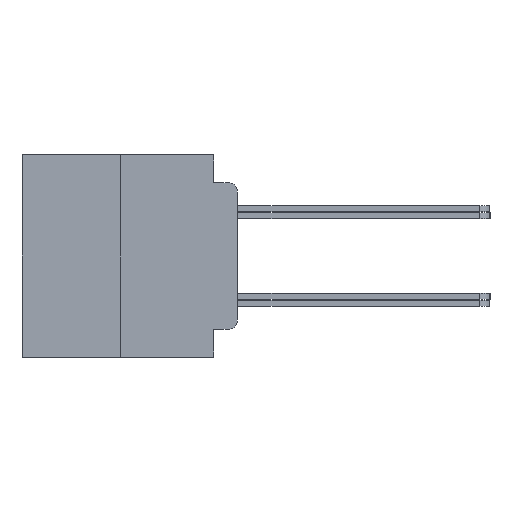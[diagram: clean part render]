
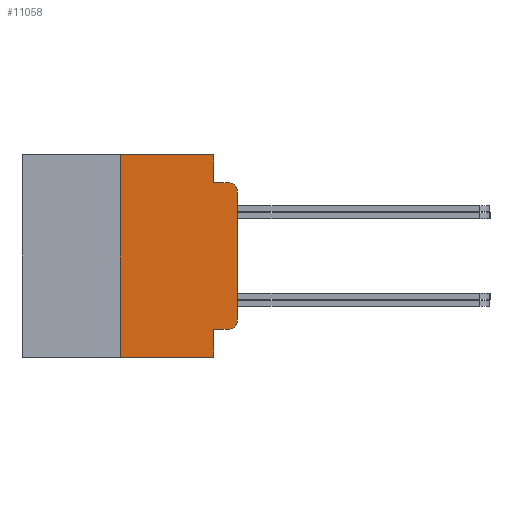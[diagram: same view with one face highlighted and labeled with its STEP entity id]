
A CAD part, left-side view. The second image highlights one B-rep face of the part: STEP entity #11058.
In plain terms, the highlighted planar face has unit normal (-1, 0, 0).
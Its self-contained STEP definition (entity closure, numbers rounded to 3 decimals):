
#409 = DIRECTION ( 'NONE',  ( 0., -1., 0. ) ) ;
#658 = VECTOR ( 'NONE', #10394, 1000. ) ;
#1171 = CARTESIAN_POINT ( 'NONE',  ( -75.603, 0.508, -3.975 ) ) ;
#1577 = PLANE ( 'NONE',  #27070 ) ;
#1828 = VERTEX_POINT ( 'NONE', #15472 ) ;
#2218 = CARTESIAN_POINT ( 'NONE',  ( -75.603, 0., -3.467 ) ) ;
#3144 = CARTESIAN_POINT ( 'NONE',  ( -75.603, 11.684, 5.486 ) ) ;
#3813 = DIRECTION ( 'NONE',  ( 0., 0., -1. ) ) ;
#3907 = DIRECTION ( 'NONE',  ( 1., 0., 0. ) ) ;
#4025 = VECTOR ( 'NONE', #7593, 1000. ) ;
#5191 = CARTESIAN_POINT ( 'NONE',  ( -75.603, 0.508, -3.467 ) ) ;
#5314 = EDGE_CURVE ( 'NONE', #27977, #28236, #26754, .T. ) ;
#5391 = FACE_OUTER_BOUND ( 'NONE', #5592, .T. ) ;
#5515 = EDGE_CURVE ( 'NONE', #28236, #13149, #27765, .T. ) ;
#5592 = EDGE_LOOP ( 'NONE', ( #6264, #5948, #16733, #16130, #12784, #23080, #10560, #15816, #26577, #27416 ) ) ;
#5948 = ORIENTED_EDGE ( 'NONE', *, *, #24408, .T. ) ;
#6264 = ORIENTED_EDGE ( 'NONE', *, *, #22663, .T. ) ;
#6413 = CARTESIAN_POINT ( 'NONE',  ( -75.603, 1.295, 5.486 ) ) ;
#6634 = LINE ( 'NONE', #12307, #8341 ) ;
#6705 = DIRECTION ( 'NONE',  ( 0., -1., 0. ) ) ;
#7097 = VERTEX_POINT ( 'NONE', #27868 ) ;
#7256 = CIRCLE ( 'NONE', #21825, 0.508 ) ;
#7593 = DIRECTION ( 'NONE',  ( 0., -1., 0. ) ) ;
#7601 = CIRCLE ( 'NONE', #17097, 0.508 ) ;
#8071 = CARTESIAN_POINT ( 'NONE',  ( -75.603, 1.295, -3.975 ) ) ;
#8266 = CARTESIAN_POINT ( 'NONE',  ( -75.603, 0.508, 3.467 ) ) ;
#8341 = VECTOR ( 'NONE', #18832, 1000. ) ;
#9638 = LINE ( 'NONE', #12302, #27867 ) ;
#10164 = VERTEX_POINT ( 'NONE', #16012 ) ;
#10394 = DIRECTION ( 'NONE',  ( 0., -1., 0. ) ) ;
#10560 = ORIENTED_EDGE ( 'NONE', *, *, #5314, .F. ) ;
#10964 = LINE ( 'NONE', #26137, #13720 ) ;
#11058 = ADVANCED_FACE ( 'NONE', ( #5391 ), #1577, .F. ) ;
#11061 = LINE ( 'NONE', #8071, #658 ) ;
#11376 = CARTESIAN_POINT ( 'NONE',  ( -75.603, 11.684, -5.486 ) ) ;
#11925 = VERTEX_POINT ( 'NONE', #2218 ) ;
#12302 = CARTESIAN_POINT ( 'NONE',  ( -75.603, 6.35, -5.486 ) ) ;
#12307 = CARTESIAN_POINT ( 'NONE',  ( -75.603, 1.295, 0. ) ) ;
#12784 = ORIENTED_EDGE ( 'NONE', *, *, #28198, .F. ) ;
#13149 = VERTEX_POINT ( 'NONE', #27766 ) ;
#13196 = EDGE_CURVE ( 'NONE', #19803, #10164, #6634, .T. ) ;
#13720 = VECTOR ( 'NONE', #21688, 1000. ) ;
#15090 = CARTESIAN_POINT ( 'NONE',  ( -75.603, 1.295, 0. ) ) ;
#15303 = LINE ( 'NONE', #22175, #27003 ) ;
#15382 = CARTESIAN_POINT ( 'NONE',  ( -75.603, 6.35, 5.486 ) ) ;
#15472 = CARTESIAN_POINT ( 'NONE',  ( -75.603, 0.508, 3.975 ) ) ;
#15816 = ORIENTED_EDGE ( 'NONE', *, *, #23272, .F. ) ;
#16012 = CARTESIAN_POINT ( 'NONE',  ( -75.603, 1.295, -5.486 ) ) ;
#16130 = ORIENTED_EDGE ( 'NONE', *, *, #22681, .T. ) ;
#16663 = EDGE_CURVE ( 'NONE', #17192, #10164, #18814, .T. ) ;
#16733 = ORIENTED_EDGE ( 'NONE', *, *, #26020, .T. ) ;
#17097 = AXIS2_PLACEMENT_3D ( 'NONE', #5191, #25015, #20584 ) ;
#17192 = VERTEX_POINT ( 'NONE', #21966 ) ;
#17288 = DIRECTION ( 'NONE',  ( 0., 0., -1. ) ) ;
#18475 = VECTOR ( 'NONE', #409, 1000. ) ;
#18806 = VERTEX_POINT ( 'NONE', #1171 ) ;
#18814 = LINE ( 'NONE', #11376, #18475 ) ;
#18831 = VECTOR ( 'NONE', #3813, 1000. ) ;
#18832 = DIRECTION ( 'NONE',  ( 0., 0., -1. ) ) ;
#19321 = DIRECTION ( 'NONE',  ( -1., 0., 0. ) ) ;
#19788 = CARTESIAN_POINT ( 'NONE',  ( -75.603, 1.295, -3.975 ) ) ;
#19803 = VERTEX_POINT ( 'NONE', #19788 ) ;
#20584 = DIRECTION ( 'NONE',  ( 0., 0., -1. ) ) ;
#21688 = DIRECTION ( 'NONE',  ( 0., 0., 1. ) ) ;
#21825 = AXIS2_PLACEMENT_3D ( 'NONE', #8266, #19321, #23755 ) ;
#21966 = CARTESIAN_POINT ( 'NONE',  ( -75.603, 6.35, -5.486 ) ) ;
#22175 = CARTESIAN_POINT ( 'NONE',  ( -75.603, 1.295, 3.975 ) ) ;
#22663 = EDGE_CURVE ( 'NONE', #19803, #18806, #11061, .T. ) ;
#22681 = EDGE_CURVE ( 'NONE', #7097, #1828, #7256, .T. ) ;
#23080 = ORIENTED_EDGE ( 'NONE', *, *, #5515, .F. ) ;
#23272 = EDGE_CURVE ( 'NONE', #17192, #27977, #9638, .T. ) ;
#23755 = DIRECTION ( 'NONE',  ( 0., 0., -1. ) ) ;
#24408 = EDGE_CURVE ( 'NONE', #18806, #11925, #7601, .T. ) ;
#25015 = DIRECTION ( 'NONE',  ( -1., 0., 0. ) ) ;
#25267 = DIRECTION ( 'NONE',  ( 0., 0., 1. ) ) ;
#26020 = EDGE_CURVE ( 'NONE', #11925, #7097, #10964, .T. ) ;
#26137 = CARTESIAN_POINT ( 'NONE',  ( -75.603, 0., 5.486 ) ) ;
#26577 = ORIENTED_EDGE ( 'NONE', *, *, #16663, .T. ) ;
#26754 = LINE ( 'NONE', #3144, #4025 ) ;
#27003 = VECTOR ( 'NONE', #6705, 1000. ) ;
#27070 = AXIS2_PLACEMENT_3D ( 'NONE', #27966, #3907, #17288 ) ;
#27416 = ORIENTED_EDGE ( 'NONE', *, *, #13196, .F. ) ;
#27765 = LINE ( 'NONE', #15090, #18831 ) ;
#27766 = CARTESIAN_POINT ( 'NONE',  ( -75.603, 1.295, 3.975 ) ) ;
#27867 = VECTOR ( 'NONE', #25267, 1000. ) ;
#27868 = CARTESIAN_POINT ( 'NONE',  ( -75.603, 0., 3.467 ) ) ;
#27966 = CARTESIAN_POINT ( 'NONE',  ( -75.603, 11.684, 5.486 ) ) ;
#27977 = VERTEX_POINT ( 'NONE', #15382 ) ;
#28198 = EDGE_CURVE ( 'NONE', #13149, #1828, #15303, .T. ) ;
#28236 = VERTEX_POINT ( 'NONE', #6413 ) ;
